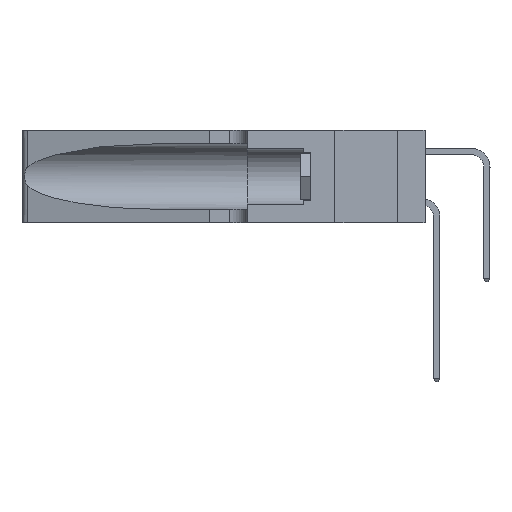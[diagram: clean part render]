
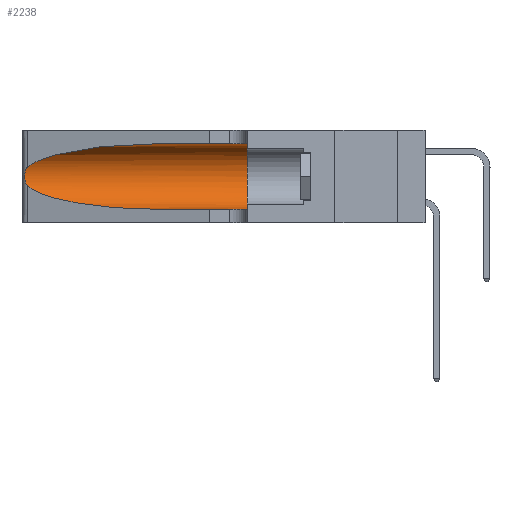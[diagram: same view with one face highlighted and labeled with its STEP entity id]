
A CAD part, left-side view. The second image highlights one B-rep face of the part: STEP entity #2238.
In plain terms, the highlighted cylindrical face has radius 3.308 mm (diameter 6.617 mm), a partial arc.
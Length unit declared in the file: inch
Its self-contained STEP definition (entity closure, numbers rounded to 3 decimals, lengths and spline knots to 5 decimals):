
#63 = EDGE_LOOP ( 'NONE', ( #15210, #18307, #1787, #22654, #1460, #22685 ) ) ;
#411 = B_SPLINE_CURVE_WITH_KNOTS ( 'NONE', 3,
 ( #1632, #17720, #5806, #19722, #7821, #21658, #9835, #23637, #11836, #25594, #13866, #1717, #15837, #3841 ),
 .UNSPECIFIED., .F., .F.,
 ( 4, 2, 2, 2, 2, 2, 4 ),
 ( 0., 0.00027, 0.00053, 0.00107, 0.0016, 0.00187, 0.00214 ),
 .UNSPECIFIED. ) ;
#594 = VERTEX_POINT ( 'NONE', #7775 ) ;
#822 = DIRECTION ( 'NONE',  ( 0., 0., -1. ) ) ;
#1460 = ORIENTED_EDGE ( 'NONE', *, *, #15396, .F. ) ;
#1632 = CARTESIAN_POINT ( 'NONE',  ( 0.25487, 1.22718, 0.22369 ) ) ;
#1717 = CARTESIAN_POINT ( 'NONE',  ( 0.25639, 1.23186, 0.15144 ) ) ;
#1787 = ORIENTED_EDGE ( 'NONE', *, *, #19797, .T. ) ;
#1987 = CARTESIAN_POINT ( 'NONE',  ( 0.1305, 0.72297, 0.31525 ) ) ;
#2238 = ADVANCED_FACE ( 'NONE', ( #24074 ), #13645, .F. ) ;
#2524 = DIRECTION ( 'NONE',  ( 0., -1., 0. ) ) ;
#2698 = CARTESIAN_POINT ( 'NONE',  ( 0.1305, 0.35, 0.31525 ) ) ;
#2895 = EDGE_CURVE ( 'NONE', #594, #4968, #10490, .T. ) ;
#3677 = CARTESIAN_POINT ( 'NONE',  ( 0.2373, 1.15595, 0.08982 ) ) ;
#3841 = CARTESIAN_POINT ( 'NONE',  ( 0.25487, 1.22718, 0.14631 ) ) ;
#4104 = CARTESIAN_POINT ( 'NONE',  ( 0.2373, 1.15595, 0.28018 ) ) ;
#4968 = VERTEX_POINT ( 'NONE', #2698 ) ;
#5806 = CARTESIAN_POINT ( 'NONE',  ( 0.25639, 1.23184, 0.21858 ) ) ;
#7063 = VERTEX_POINT ( 'NONE', #19317 ) ;
#7762 = CARTESIAN_POINT ( 'NONE',  ( 0.25487, 1.22718, 0.14631 ) ) ;
#7775 = CARTESIAN_POINT ( 'NONE',  ( 0.1305, 0.72297, 0.31525 ) ) ;
#7821 = CARTESIAN_POINT ( 'NONE',  ( 0.25854, 1.2359, 0.20912 ) ) ;
#7896 = DIRECTION ( 'NONE',  ( 0., 1., 0. ) ) ;
#8310 = EDGE_CURVE ( 'NONE', #15582, #14136, #17668, .T. ) ;
#8343 = AXIS2_PLACEMENT_3D ( 'NONE', #14996, #13000, #822 ) ;
#8843 = CARTESIAN_POINT ( 'NONE',  ( 0.1305, 1.61858, 0.31525 ) ) ;
#9383 = AXIS2_PLACEMENT_3D ( 'NONE', #19796, #7896, #21722 ) ;
#9711 = CARTESIAN_POINT ( 'NONE',  ( 0.25487, 1.22718, 0.14631 ) ) ;
#9835 = CARTESIAN_POINT ( 'NONE',  ( 0.26075, 1.23896, 0.19203 ) ) ;
#9963 = EDGE_CURVE ( 'NONE', #7063, #19124, #411, .T. ) ;
#10047 = EDGE_CURVE ( 'NONE', #594, #7063, #21770, .T. ) ;
#10490 = LINE ( 'NONE', #8843, #25567 ) ;
#10721 =( BOUNDED_CURVE ( )  B_SPLINE_CURVE ( 3, ( #7762, #3677, #25533, #13809 ),
 .UNSPECIFIED., .F., .T. ) 
 B_SPLINE_CURVE_WITH_KNOTS ( ( 4, 4 ),
 ( 3.44316, 4.71239 ),
 .UNSPECIFIED. ) 
 CURVE ( )  GEOMETRIC_REPRESENTATION_ITEM ( )  RATIONAL_B_SPLINE_CURVE ( ( 1., 0.87, 0.87, 1. ) ) 
 REPRESENTATION_ITEM ( '' )  );
#10857 = DIRECTION ( 'NONE',  ( 0., -1., 0. ) ) ;
#11836 = CARTESIAN_POINT ( 'NONE',  ( 0.26017, 1.23833, 0.17102 ) ) ;
#12612 = CARTESIAN_POINT ( 'NONE',  ( 0.1305, 1.61858, 0.05475 ) ) ;
#13000 = DIRECTION ( 'NONE',  ( 0., -1., 0. ) ) ;
#13512 = CIRCLE ( 'NONE', #9383, 0.13025 ) ;
#13645 = CYLINDRICAL_SURFACE ( 'NONE', #8343, 0.13025 ) ;
#13809 = CARTESIAN_POINT ( 'NONE',  ( 0.1305, 0.72297, 0.05475 ) ) ;
#13866 = CARTESIAN_POINT ( 'NONE',  ( 0.25789, 1.23486, 0.15765 ) ) ;
#14136 = VERTEX_POINT ( 'NONE', #25712 ) ;
#14996 = CARTESIAN_POINT ( 'NONE',  ( 0.1305, 1.61858, 0.185 ) ) ;
#15210 = ORIENTED_EDGE ( 'NONE', *, *, #10047, .T. ) ;
#15396 = EDGE_CURVE ( 'NONE', #4968, #14136, #13512, .T. ) ;
#15582 = VERTEX_POINT ( 'NONE', #18771 ) ;
#15837 = CARTESIAN_POINT ( 'NONE',  ( 0.25555, 1.22993, 0.14849 ) ) ;
#17064 = VECTOR ( 'NONE', #2524, 39.37008 ) ;
#17668 = LINE ( 'NONE', #12612, #17064 ) ;
#17720 = CARTESIAN_POINT ( 'NONE',  ( 0.25555, 1.22994, 0.2215 ) ) ;
#18072 = CARTESIAN_POINT ( 'NONE',  ( 0.25487, 1.22718, 0.22369 ) ) ;
#18307 = ORIENTED_EDGE ( 'NONE', *, *, #9963, .T. ) ;
#18771 = CARTESIAN_POINT ( 'NONE',  ( 0.1305, 0.72297, 0.05475 ) ) ;
#19124 = VERTEX_POINT ( 'NONE', #9711 ) ;
#19317 = CARTESIAN_POINT ( 'NONE',  ( 0.25487, 1.22718, 0.22369 ) ) ;
#19722 = CARTESIAN_POINT ( 'NONE',  ( 0.25787, 1.23484, 0.2124 ) ) ;
#19796 = CARTESIAN_POINT ( 'NONE',  ( 0.1305, 0.35, 0.185 ) ) ;
#19797 = EDGE_CURVE ( 'NONE', #19124, #15582, #10721, .T. ) ;
#21658 = CARTESIAN_POINT ( 'NONE',  ( 0.26018, 1.23835, 0.19895 ) ) ;
#21722 = DIRECTION ( 'NONE',  ( 0., 0., 1. ) ) ;
#21770 =( BOUNDED_CURVE ( )  B_SPLINE_CURVE ( 3, ( #1987, #25841, #4104, #18072 ),
 .UNSPECIFIED., .F., .F. ) 
 B_SPLINE_CURVE_WITH_KNOTS ( ( 4, 4 ),
 ( 1.5708, 2.84003 ),
 .UNSPECIFIED. ) 
 CURVE ( )  GEOMETRIC_REPRESENTATION_ITEM ( )  RATIONAL_B_SPLINE_CURVE ( ( 1., 0.87, 0.87, 1. ) ) 
 REPRESENTATION_ITEM ( '' )  );
#22654 = ORIENTED_EDGE ( 'NONE', *, *, #8310, .T. ) ;
#22685 = ORIENTED_EDGE ( 'NONE', *, *, #2895, .F. ) ;
#23637 = CARTESIAN_POINT ( 'NONE',  ( 0.26075, 1.23896, 0.178 ) ) ;
#24074 = FACE_OUTER_BOUND ( 'NONE', #63, .T. ) ;
#25533 = CARTESIAN_POINT ( 'NONE',  ( 0.18966, 0.96281, 0.05475 ) ) ;
#25567 = VECTOR ( 'NONE', #10857, 39.37008 ) ;
#25594 = CARTESIAN_POINT ( 'NONE',  ( 0.25856, 1.23593, 0.16098 ) ) ;
#25712 = CARTESIAN_POINT ( 'NONE',  ( 0.1305, 0.35, 0.05475 ) ) ;
#25841 = CARTESIAN_POINT ( 'NONE',  ( 0.18966, 0.96281, 0.31525 ) ) ;
